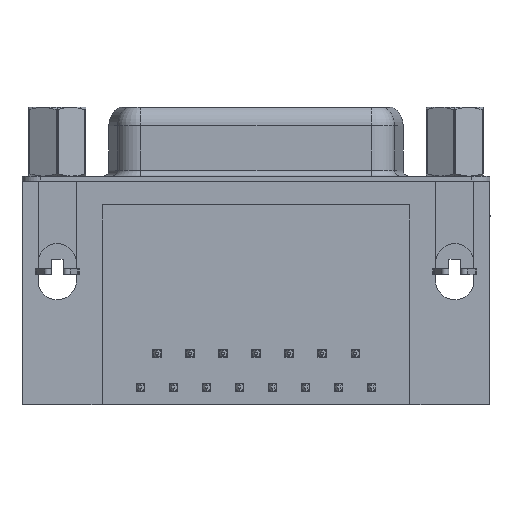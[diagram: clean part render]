
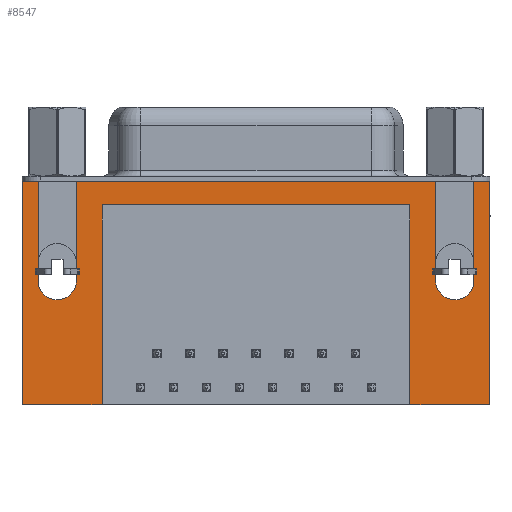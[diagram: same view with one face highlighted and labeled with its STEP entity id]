
A CAD part, front view. The second image highlights one B-rep face of the part: STEP entity #8547.
In plain terms, the highlighted planar face has unit normal (0, -1, 0).
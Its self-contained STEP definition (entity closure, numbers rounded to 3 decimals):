
#166 = LINE ( 'NONE', #1275, #9517 ) ;
#218 = CARTESIAN_POINT ( 'NONE',  ( 29.555, -6.275, -2. ) ) ;
#227 = ORIENTED_EDGE ( 'NONE', *, *, #27186, .F. ) ;
#635 = VERTEX_POINT ( 'NONE', #17222 ) ;
#737 = LINE ( 'NONE', #13694, #2208 ) ;
#784 = DIRECTION ( 'NONE',  ( 0., -1., 0. ) ) ;
#1131 = EDGE_LOOP ( 'NONE', ( #20213, #23170, #22368, #227, #7712, #21269, #21749, #2039, #21244, #10385, #6762, #26909, #28129, #13001, #25608, #14261 ) ) ;
#1275 = CARTESIAN_POINT ( 'NONE',  ( -2.935, -6.275, 0. ) ) ;
#2039 = ORIENTED_EDGE ( 'NONE', *, *, #9593, .F. ) ;
#2208 = VECTOR ( 'NONE', #18287, 1000. ) ;
#2313 = VECTOR ( 'NONE', #8041, 1000. ) ;
#2344 = LINE ( 'NONE', #16796, #2313 ) ;
#2382 = CIRCLE ( 'NONE', #12424, 1.6 ) ;
#3166 = LINE ( 'NONE', #20351, #3295 ) ;
#3295 = VECTOR ( 'NONE', #6986, 1000. ) ;
#3311 = VERTEX_POINT ( 'NONE', #28221 ) ;
#4174 = FACE_OUTER_BOUND ( 'NONE', #1131, .T. ) ;
#4420 = EDGE_CURVE ( 'NONE', #24480, #17876, #21884, .T. ) ;
#4448 = VERTEX_POINT ( 'NONE', #17974 ) ;
#4814 = VERTEX_POINT ( 'NONE', #13015 ) ;
#5377 = CARTESIAN_POINT ( 'NONE',  ( 3.765, -6.275, -2. ) ) ;
#5681 = CARTESIAN_POINT ( 'NONE',  ( 33.32, -6.275, -8.35 ) ) ;
#5885 = CARTESIAN_POINT ( 'NONE',  ( -2.935, -6.275, 0. ) ) ;
#6240 = CARTESIAN_POINT ( 'NONE',  ( 34.92, -6.275, 0. ) ) ;
#6715 = EDGE_CURVE ( 'NONE', #635, #13092, #11724, .T. ) ;
#6762 = ORIENTED_EDGE ( 'NONE', *, *, #15634, .F. ) ;
#6981 = DIRECTION ( 'NONE',  ( -1., 0., 0. ) ) ;
#6986 = DIRECTION ( 'NONE',  ( 0., 0., -1. ) ) ;
#7286 = PLANE ( 'NONE',  #14236 ) ;
#7350 = CARTESIAN_POINT ( 'NONE',  ( -2.935, -6.275, -2.5 ) ) ;
#7712 = ORIENTED_EDGE ( 'NONE', *, *, #4420, .F. ) ;
#7839 = DIRECTION ( 'NONE',  ( -1., 0., 0. ) ) ;
#7924 = VERTEX_POINT ( 'NONE', #9327 ) ;
#8025 = DIRECTION ( 'NONE',  ( 0., 0., -1. ) ) ;
#8041 = DIRECTION ( 'NONE',  ( 0., 0., -1. ) ) ;
#8208 = DIRECTION ( 'NONE',  ( -1., 0., 0. ) ) ;
#8273 = CARTESIAN_POINT ( 'NONE',  ( 1.6, -6.275, -8.35 ) ) ;
#8547 = ADVANCED_FACE ( 'NONE', ( #4174 ), #7286, .T. ) ;
#9327 = CARTESIAN_POINT ( 'NONE',  ( -1.6, -6.275, 0. ) ) ;
#9365 = CARTESIAN_POINT ( 'NONE',  ( 31.72, -6.275, -8.35 ) ) ;
#9496 = DIRECTION ( 'NONE',  ( 0., 0., -1. ) ) ;
#9517 = VECTOR ( 'NONE', #12122, 1000. ) ;
#9593 = EDGE_CURVE ( 'NONE', #25589, #7924, #27963, .T. ) ;
#9630 = EDGE_CURVE ( 'NONE', #3311, #635, #27874, .T. ) ;
#9730 = CARTESIAN_POINT ( 'NONE',  ( 0., -6.275, -8.35 ) ) ;
#10196 = EDGE_CURVE ( 'NONE', #7924, #27295, #25211, .T. ) ;
#10236 = CARTESIAN_POINT ( 'NONE',  ( -1.6, -6.275, 0. ) ) ;
#10385 = ORIENTED_EDGE ( 'NONE', *, *, #26826, .F. ) ;
#10582 = DIRECTION ( 'NONE',  ( 0., 0., 1. ) ) ;
#10644 = CARTESIAN_POINT ( 'NONE',  ( 1.6, -6.275, 0. ) ) ;
#11321 = LINE ( 'NONE', #5885, #14273 ) ;
#11683 = VECTOR ( 'NONE', #8208, 1000. ) ;
#11724 = LINE ( 'NONE', #16550, #11683 ) ;
#11934 = CARTESIAN_POINT ( 'NONE',  ( 36.255, -6.275, 0. ) ) ;
#11948 = DIRECTION ( 'NONE',  ( 1., 0., 0. ) ) ;
#12122 = DIRECTION ( 'NONE',  ( 1., 0., 0. ) ) ;
#12221 = EDGE_CURVE ( 'NONE', #20446, #18660, #16829, .T. ) ;
#12424 = AXIS2_PLACEMENT_3D ( 'NONE', #5681, #21195, #7839 ) ;
#12791 = CARTESIAN_POINT ( 'NONE',  ( 34.92, -6.275, 0. ) ) ;
#12894 = LINE ( 'NONE', #7350, #27386 ) ;
#13001 = ORIENTED_EDGE ( 'NONE', *, *, #24693, .F. ) ;
#13015 = CARTESIAN_POINT ( 'NONE',  ( -2.935, -6.275, -18.76 ) ) ;
#13092 = VERTEX_POINT ( 'NONE', #5377 ) ;
#13362 = DIRECTION ( 'NONE',  ( 0., 0., 1. ) ) ;
#13459 = CARTESIAN_POINT ( 'NONE',  ( -2.935, -6.275, 0. ) ) ;
#13694 = CARTESIAN_POINT ( 'NONE',  ( 36.255, -6.275, -18.76 ) ) ;
#14236 = AXIS2_PLACEMENT_3D ( 'NONE', #18382, #784, #9496 ) ;
#14261 = ORIENTED_EDGE ( 'NONE', *, *, #25929, .F. ) ;
#14273 = VECTOR ( 'NONE', #19142, 1000. ) ;
#14659 = LINE ( 'NONE', #22591, #19739 ) ;
#14882 = VERTEX_POINT ( 'NONE', #22044 ) ;
#15245 = AXIS2_PLACEMENT_3D ( 'NONE', #9730, #25470, #11948 ) ;
#15417 = CARTESIAN_POINT ( 'NONE',  ( -1.6, -6.275, -8.35 ) ) ;
#15507 = CARTESIAN_POINT ( 'NONE',  ( -2.935, -6.275, 0. ) ) ;
#15634 = EDGE_CURVE ( 'NONE', #13092, #14882, #3166, .T. ) ;
#16550 = CARTESIAN_POINT ( 'NONE',  ( 3.765, -6.275, -2. ) ) ;
#16796 = CARTESIAN_POINT ( 'NONE',  ( 31.72, -6.275, 0. ) ) ;
#16829 = LINE ( 'NONE', #6240, #16981 ) ;
#16981 = VECTOR ( 'NONE', #21580, 1000. ) ;
#17216 = CARTESIAN_POINT ( 'NONE',  ( 34.92, -6.275, -8.35 ) ) ;
#17222 = CARTESIAN_POINT ( 'NONE',  ( 29.555, -6.275, -2. ) ) ;
#17311 = EDGE_CURVE ( 'NONE', #4448, #22626, #24464, .T. ) ;
#17752 = DIRECTION ( 'NONE',  ( 1., 0., 0. ) ) ;
#17876 = VERTEX_POINT ( 'NONE', #27564 ) ;
#17974 = CARTESIAN_POINT ( 'NONE',  ( 36.255, -6.275, -18.76 ) ) ;
#18287 = DIRECTION ( 'NONE',  ( -1., 0., 0. ) ) ;
#18382 = CARTESIAN_POINT ( 'NONE',  ( -2.935, -6.275, -2.5 ) ) ;
#18660 = VERTEX_POINT ( 'NONE', #12791 ) ;
#19142 = DIRECTION ( 'NONE',  ( 1., 0., 0. ) ) ;
#19739 = VECTOR ( 'NONE', #6981, 1000. ) ;
#20213 = ORIENTED_EDGE ( 'NONE', *, *, #12221, .F. ) ;
#20351 = CARTESIAN_POINT ( 'NONE',  ( 3.765, -6.275, -2. ) ) ;
#20446 = VERTEX_POINT ( 'NONE', #17216 ) ;
#21195 = DIRECTION ( 'NONE',  ( 0., -1., 0. ) ) ;
#21244 = ORIENTED_EDGE ( 'NONE', *, *, #23891, .F. ) ;
#21269 = ORIENTED_EDGE ( 'NONE', *, *, #23975, .F. ) ;
#21580 = DIRECTION ( 'NONE',  ( 0., 0., 1. ) ) ;
#21653 = VECTOR ( 'NONE', #10582, 1000. ) ;
#21749 = ORIENTED_EDGE ( 'NONE', *, *, #10196, .F. ) ;
#21884 = LINE ( 'NONE', #10644, #21653 ) ;
#22044 = CARTESIAN_POINT ( 'NONE',  ( 3.765, -6.275, -18.76 ) ) ;
#22186 = EDGE_CURVE ( 'NONE', #27166, #23875, #2344, .T. ) ;
#22368 = ORIENTED_EDGE ( 'NONE', *, *, #22186, .F. ) ;
#22591 = CARTESIAN_POINT ( 'NONE',  ( 36.255, -6.275, -18.76 ) ) ;
#22626 = VERTEX_POINT ( 'NONE', #11934 ) ;
#22649 = DIRECTION ( 'NONE',  ( 0., 0., 1. ) ) ;
#22941 = DIRECTION ( 'NONE',  ( 0., 0., 1. ) ) ;
#23170 = ORIENTED_EDGE ( 'NONE', *, *, #26772, .F. ) ;
#23559 = CARTESIAN_POINT ( 'NONE',  ( 31.72, -6.275, 0. ) ) ;
#23875 = VERTEX_POINT ( 'NONE', #9365 ) ;
#23891 = EDGE_CURVE ( 'NONE', #4814, #25589, #12894, .T. ) ;
#23975 = EDGE_CURVE ( 'NONE', #27295, #24480, #26886, .T. ) ;
#24227 = VECTOR ( 'NONE', #22649, 1000. ) ;
#24464 = LINE ( 'NONE', #27305, #24227 ) ;
#24480 = VERTEX_POINT ( 'NONE', #8273 ) ;
#24693 = EDGE_CURVE ( 'NONE', #4448, #3311, #737, .T. ) ;
#25211 = LINE ( 'NONE', #10236, #25268 ) ;
#25268 = VECTOR ( 'NONE', #8025, 1000. ) ;
#25470 = DIRECTION ( 'NONE',  ( 0., -1., 0. ) ) ;
#25589 = VERTEX_POINT ( 'NONE', #13459 ) ;
#25608 = ORIENTED_EDGE ( 'NONE', *, *, #17311, .T. ) ;
#25929 = EDGE_CURVE ( 'NONE', #18660, #22626, #166, .T. ) ;
#26772 = EDGE_CURVE ( 'NONE', #23875, #20446, #2382, .T. ) ;
#26826 = EDGE_CURVE ( 'NONE', #14882, #4814, #14659, .T. ) ;
#26886 = CIRCLE ( 'NONE', #15245, 1.6 ) ;
#26909 = ORIENTED_EDGE ( 'NONE', *, *, #6715, .F. ) ;
#27166 = VERTEX_POINT ( 'NONE', #23559 ) ;
#27186 = EDGE_CURVE ( 'NONE', #17876, #27166, #11321, .T. ) ;
#27295 = VERTEX_POINT ( 'NONE', #15417 ) ;
#27305 = CARTESIAN_POINT ( 'NONE',  ( 36.255, -6.275, -2.5 ) ) ;
#27386 = VECTOR ( 'NONE', #22941, 1000. ) ;
#27564 = CARTESIAN_POINT ( 'NONE',  ( 1.6, -6.275, 0. ) ) ;
#27874 = LINE ( 'NONE', #218, #27933 ) ;
#27905 = VECTOR ( 'NONE', #17752, 1000. ) ;
#27933 = VECTOR ( 'NONE', #13362, 1000. ) ;
#27963 = LINE ( 'NONE', #15507, #27905 ) ;
#28129 = ORIENTED_EDGE ( 'NONE', *, *, #9630, .F. ) ;
#28221 = CARTESIAN_POINT ( 'NONE',  ( 29.555, -6.275, -18.76 ) ) ;
